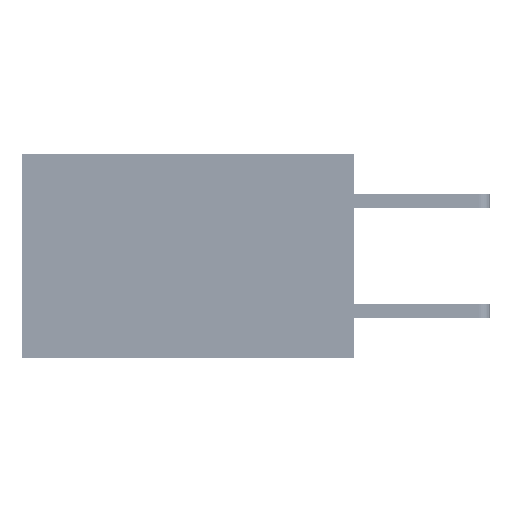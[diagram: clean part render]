
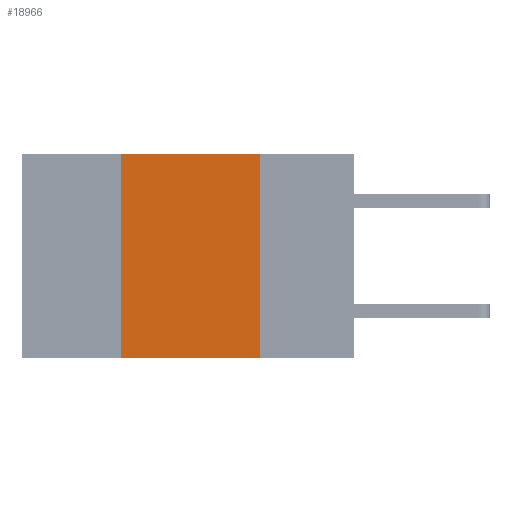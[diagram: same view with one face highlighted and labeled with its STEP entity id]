
A CAD part, left-side view. The second image highlights one B-rep face of the part: STEP entity #18966.
In plain terms, the highlighted planar face has unit normal (-1, 0, 0).
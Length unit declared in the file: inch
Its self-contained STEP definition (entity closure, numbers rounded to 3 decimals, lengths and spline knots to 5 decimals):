
#443 = CARTESIAN_POINT ( 'NONE',  ( 0., 0.42, 0. ) ) ;
#4112 = EDGE_LOOP ( 'NONE', ( #19039, #24165, #26257, #31865 ) ) ;
#4753 = CARTESIAN_POINT ( 'NONE',  ( 0., 0.6, 0. ) ) ;
#8821 = LINE ( 'NONE', #17817, #46953 ) ;
#10880 = CARTESIAN_POINT ( 'NONE',  ( 0., 0.42, 0. ) ) ;
#11052 = DIRECTION ( 'NONE',  ( 0., -1., 0. ) ) ;
#11750 = CARTESIAN_POINT ( 'NONE',  ( 0., 0.42, -0.37 ) ) ;
#11984 = DIRECTION ( 'NONE',  ( 0., -1., 0. ) ) ;
#14030 = EDGE_CURVE ( 'NONE', #18207, #23029, #8821, .T. ) ;
#14695 = CARTESIAN_POINT ( 'NONE',  ( 0., 0.17, -0.37 ) ) ;
#17817 = CARTESIAN_POINT ( 'NONE',  ( 0., 0.6, 0. ) ) ;
#18207 = VERTEX_POINT ( 'NONE', #443 ) ;
#18966 = ADVANCED_FACE ( 'NONE', ( #37216 ), #34174, .F. ) ;
#19039 = ORIENTED_EDGE ( 'NONE', *, *, #37076, .F. ) ;
#20538 = LINE ( 'NONE', #37521, #47704 ) ;
#23029 = VERTEX_POINT ( 'NONE', #45554 ) ;
#23873 = AXIS2_PLACEMENT_3D ( 'NONE', #4753, #34330, #41922 ) ;
#24165 = ORIENTED_EDGE ( 'NONE', *, *, #14030, .F. ) ;
#24174 = EDGE_CURVE ( 'NONE', #28981, #18207, #39357, .T. ) ;
#26257 = ORIENTED_EDGE ( 'NONE', *, *, #24174, .F. ) ;
#26705 = CARTESIAN_POINT ( 'NONE',  ( 0., 0.6, -0.37 ) ) ;
#28981 = VERTEX_POINT ( 'NONE', #11750 ) ;
#29714 = LINE ( 'NONE', #26705, #35516 ) ;
#31720 = VERTEX_POINT ( 'NONE', #14695 ) ;
#31865 = ORIENTED_EDGE ( 'NONE', *, *, #38771, .T. ) ;
#34174 = PLANE ( 'NONE',  #23873 ) ;
#34330 = DIRECTION ( 'NONE',  ( 1., 0., 0. ) ) ;
#35516 = VECTOR ( 'NONE', #11984, 39.37008 ) ;
#35843 = VECTOR ( 'NONE', #36773, 39.37008 ) ;
#36773 = DIRECTION ( 'NONE',  ( 0., 0., 1. ) ) ;
#37076 = EDGE_CURVE ( 'NONE', #23029, #31720, #20538, .T. ) ;
#37216 = FACE_OUTER_BOUND ( 'NONE', #4112, .T. ) ;
#37521 = CARTESIAN_POINT ( 'NONE',  ( 0., 0.17, 0. ) ) ;
#38771 = EDGE_CURVE ( 'NONE', #28981, #31720, #29714, .T. ) ;
#39357 = LINE ( 'NONE', #10880, #35843 ) ;
#41922 = DIRECTION ( 'NONE',  ( 0., 0., -1. ) ) ;
#44927 = DIRECTION ( 'NONE',  ( 0., 0., -1. ) ) ;
#45554 = CARTESIAN_POINT ( 'NONE',  ( 0., 0.17, 0. ) ) ;
#46953 = VECTOR ( 'NONE', #11052, 39.37008 ) ;
#47704 = VECTOR ( 'NONE', #44927, 39.37008 ) ;
